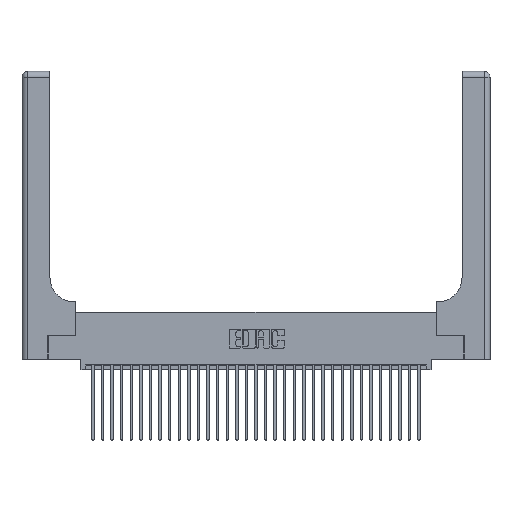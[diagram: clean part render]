
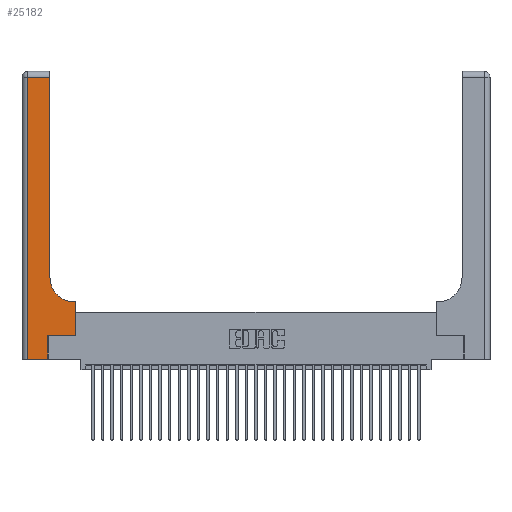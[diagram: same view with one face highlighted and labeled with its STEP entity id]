
A CAD part, top view. The second image highlights one B-rep face of the part: STEP entity #25182.
In plain terms, the highlighted planar face has unit normal (0, 0, 1).
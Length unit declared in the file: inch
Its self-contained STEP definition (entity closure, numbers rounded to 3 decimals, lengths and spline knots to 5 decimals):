
#134 = VERTEX_POINT ( 'NONE', #9074 ) ;
#1716 = DIRECTION ( 'NONE',  ( 1., 0., 0. ) ) ;
#1900 = CARTESIAN_POINT ( 'NONE',  ( 0.2915, 3., 0.37 ) ) ;
#2075 = EDGE_CURVE ( 'NONE', #31205, #22011, #28269, .T. ) ;
#2363 = VECTOR ( 'NONE', #30615, 39.37008 ) ;
#2448 = DIRECTION ( 'NONE',  ( 0., 0., -1. ) ) ;
#2728 = CARTESIAN_POINT ( 'NONE',  ( 0.06, 2.94, 0.37 ) ) ;
#3565 = ORIENTED_EDGE ( 'NONE', *, *, #27817, .T. ) ;
#3765 = VECTOR ( 'NONE', #30601, 39.37008 ) ;
#3968 = CARTESIAN_POINT ( 'NONE',  ( 0.2915, 0.6, 0.37 ) ) ;
#5168 = ORIENTED_EDGE ( 'NONE', *, *, #2075, .T. ) ;
#5182 = PLANE ( 'NONE',  #18170 ) ;
#5594 = ORIENTED_EDGE ( 'NONE', *, *, #10091, .T. ) ;
#7389 = VECTOR ( 'NONE', #28058, 39.37008 ) ;
#7474 = VECTOR ( 'NONE', #10202, 39.37008 ) ;
#7548 = EDGE_CURVE ( 'NONE', #22011, #11753, #13620, .T. ) ;
#7840 = DIRECTION ( 'NONE',  ( -1., 0., 0. ) ) ;
#8225 = EDGE_LOOP ( 'NONE', ( #26803, #27267, #23375, #26622, #3565, #5168, #9538, #9730, #5594 ) ) ;
#8520 = AXIS2_PLACEMENT_3D ( 'NONE', #30445, #28249, #25972 ) ;
#9074 = CARTESIAN_POINT ( 'NONE',  ( 0.2915, 2.94, 0.37 ) ) ;
#9538 = ORIENTED_EDGE ( 'NONE', *, *, #7548, .T. ) ;
#9730 = ORIENTED_EDGE ( 'NONE', *, *, #16797, .T. ) ;
#10091 = EDGE_CURVE ( 'NONE', #21469, #18599, #21007, .T. ) ;
#10202 = DIRECTION ( 'NONE',  ( 1., 0., 0. ) ) ;
#10238 = VECTOR ( 'NONE', #28587, 39.37008 ) ;
#10465 = VECTOR ( 'NONE', #27227, 39.37008 ) ;
#10847 = CARTESIAN_POINT ( 'NONE',  ( 0.06, 0., 0.37 ) ) ;
#11627 = FACE_OUTER_BOUND ( 'NONE', #8225, .T. ) ;
#11753 = VERTEX_POINT ( 'NONE', #24792 ) ;
#11828 = VERTEX_POINT ( 'NONE', #14115 ) ;
#12162 = EDGE_CURVE ( 'NONE', #12192, #13875, #15624, .T. ) ;
#12192 = VERTEX_POINT ( 'NONE', #2728 ) ;
#12835 = EDGE_CURVE ( 'NONE', #134, #12192, #24064, .T. ) ;
#13620 = LINE ( 'NONE', #25606, #3765 ) ;
#13722 = CARTESIAN_POINT ( 'NONE',  ( 0.269, 0., 0.37 ) ) ;
#13875 = VERTEX_POINT ( 'NONE', #10847 ) ;
#13896 = LINE ( 'NONE', #13722, #25292 ) ;
#14115 = CARTESIAN_POINT ( 'NONE',  ( 0.269, 0., 0.37 ) ) ;
#14321 = EDGE_CURVE ( 'NONE', #18599, #134, #28490, .T. ) ;
#14792 = CARTESIAN_POINT ( 'NONE',  ( 0.269, 0.25, 0.37 ) ) ;
#15624 = LINE ( 'NONE', #30800, #7389 ) ;
#16248 = DIRECTION ( 'NONE',  ( 0., 1., 0. ) ) ;
#16797 = EDGE_CURVE ( 'NONE', #11753, #21469, #20670, .T. ) ;
#18170 = AXIS2_PLACEMENT_3D ( 'NONE', #33691, #2448, #7840 ) ;
#18599 = VERTEX_POINT ( 'NONE', #26870 ) ;
#19233 = EDGE_CURVE ( 'NONE', #13875, #11828, #29886, .T. ) ;
#20670 = LINE ( 'NONE', #3968, #10465 ) ;
#21007 = CIRCLE ( 'NONE', #8520, 0.25 ) ;
#21469 = VERTEX_POINT ( 'NONE', #31691 ) ;
#22011 = VERTEX_POINT ( 'NONE', #31313 ) ;
#23355 = CARTESIAN_POINT ( 'NONE',  ( 0., 2.94, 0.37 ) ) ;
#23375 = ORIENTED_EDGE ( 'NONE', *, *, #12162, .T. ) ;
#24064 = LINE ( 'NONE', #23355, #10238 ) ;
#24792 = CARTESIAN_POINT ( 'NONE',  ( 0.5585, 0.6, 0.37 ) ) ;
#25182 = ADVANCED_FACE ( 'NONE', ( #11627 ), #5182, .F. ) ;
#25292 = VECTOR ( 'NONE', #16248, 39.37008 ) ;
#25606 = CARTESIAN_POINT ( 'NONE',  ( 0.5585, 0.25, 0.37 ) ) ;
#25822 = VECTOR ( 'NONE', #1716, 39.37008 ) ;
#25972 = DIRECTION ( 'NONE',  ( 1., 0., 0. ) ) ;
#26622 = ORIENTED_EDGE ( 'NONE', *, *, #19233, .T. ) ;
#26803 = ORIENTED_EDGE ( 'NONE', *, *, #14321, .T. ) ;
#26870 = CARTESIAN_POINT ( 'NONE',  ( 0.2915, 0.85, 0.37 ) ) ;
#27227 = DIRECTION ( 'NONE',  ( -1., 0., 0. ) ) ;
#27267 = ORIENTED_EDGE ( 'NONE', *, *, #12835, .T. ) ;
#27817 = EDGE_CURVE ( 'NONE', #11828, #31205, #13896, .T. ) ;
#28058 = DIRECTION ( 'NONE',  ( 0., -1., 0. ) ) ;
#28249 = DIRECTION ( 'NONE',  ( 0., 0., -1. ) ) ;
#28269 = LINE ( 'NONE', #14792, #25822 ) ;
#28490 = LINE ( 'NONE', #1900, #2363 ) ;
#28587 = DIRECTION ( 'NONE',  ( -1., 0., 0. ) ) ;
#29884 = CARTESIAN_POINT ( 'NONE',  ( 0., 0., 0.37 ) ) ;
#29886 = LINE ( 'NONE', #29884, #7474 ) ;
#30445 = CARTESIAN_POINT ( 'NONE',  ( 0.5415, 0.85, 0.37 ) ) ;
#30601 = DIRECTION ( 'NONE',  ( 0., 1., 0. ) ) ;
#30615 = DIRECTION ( 'NONE',  ( 0., 1., 0. ) ) ;
#30800 = CARTESIAN_POINT ( 'NONE',  ( 0.06, 3., 0.37 ) ) ;
#31205 = VERTEX_POINT ( 'NONE', #31655 ) ;
#31313 = CARTESIAN_POINT ( 'NONE',  ( 0.5585, 0.25, 0.37 ) ) ;
#31655 = CARTESIAN_POINT ( 'NONE',  ( 0.269, 0.25, 0.37 ) ) ;
#31691 = CARTESIAN_POINT ( 'NONE',  ( 0.5415, 0.6, 0.37 ) ) ;
#33691 = CARTESIAN_POINT ( 'NONE',  ( 0., 3., 0.37 ) ) ;
